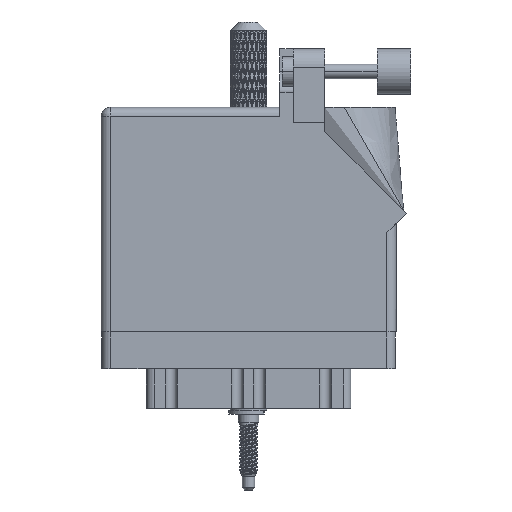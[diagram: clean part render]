
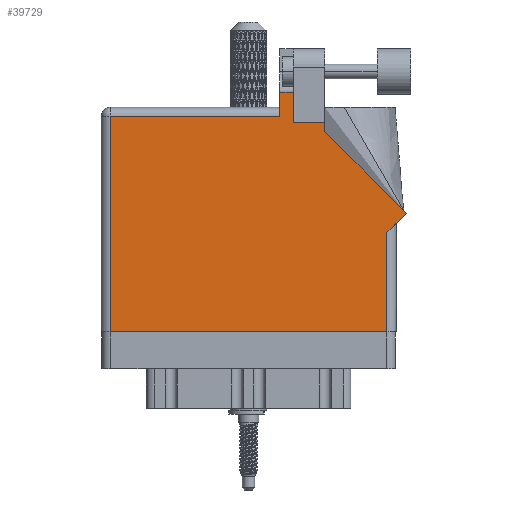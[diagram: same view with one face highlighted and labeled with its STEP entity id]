
A CAD part, front view. The second image highlights one B-rep face of the part: STEP entity #39729.
In plain terms, the highlighted face is planar.
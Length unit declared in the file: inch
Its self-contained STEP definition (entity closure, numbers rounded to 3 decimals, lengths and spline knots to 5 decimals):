
#113 = VECTOR ( 'NONE', #100295, 39.37008 ) ;
#389 = CARTESIAN_POINT ( 'NONE',  ( 1.217, 1.6315, 0. ) ) ;
#774 = ORIENTED_EDGE ( 'NONE', *, *, #37043, .T. ) ;
#975 = DIRECTION ( 'NONE',  ( 0., -1., 0. ) ) ;
#2414 = VERTEX_POINT ( 'NONE', #103825 ) ;
#4596 = ORIENTED_EDGE ( 'NONE', *, *, #92486, .T. ) ;
#6521 = VERTEX_POINT ( 'NONE', #102149 ) ;
#6803 = ORIENTED_EDGE ( 'NONE', *, *, #50928, .T. ) ;
#7591 = VERTEX_POINT ( 'NONE', #65473 ) ;
#9100 = VECTOR ( 'NONE', #975, 39.37008 ) ;
#10269 = ORIENTED_EDGE ( 'NONE', *, *, #17523, .T. ) ;
#11165 = EDGE_CURVE ( 'NONE', #44501, #67315, #84320, .T. ) ;
#11763 = CARTESIAN_POINT ( 'NONE',  ( 1.524, 1.36442, 0. ) ) ;
#12683 = FACE_OUTER_BOUND ( 'NONE', #38110, .T. ) ;
#12820 = LINE ( 'NONE', #21805, #57870 ) ;
#13620 = CARTESIAN_POINT ( 'NONE',  ( 1.217, 1.53, 0. ) ) ;
#16835 = DIRECTION ( 'NONE',  ( 0., 1., 0. ) ) ;
#17523 = EDGE_CURVE ( 'NONE', #102263, #36767, #73571, .T. ) ;
#19213 = CARTESIAN_POINT ( 'NONE',  ( 0., 1.468, 0. ) ) ;
#21202 = CARTESIAN_POINT ( 'NONE',  ( 2.01, 0.737, 0. ) ) ;
#21805 = CARTESIAN_POINT ( 'NONE',  ( 0., 0., 0. ) ) ;
#22273 = VERTEX_POINT ( 'NONE', #91431 ) ;
#22643 = VERTEX_POINT ( 'NONE', #88695 ) ;
#23249 = EDGE_CURVE ( 'NONE', #51740, #22273, #95242, .T. ) ;
#23280 = CARTESIAN_POINT ( 'NONE',  ( 2.08071, 0.80771, 0. ) ) ;
#23488 = VECTOR ( 'NONE', #25501, 39.37008 ) ;
#25501 = DIRECTION ( 'NONE',  ( -1., 0., 0. ) ) ;
#25826 = VECTOR ( 'NONE', #86325, 39.37008 ) ;
#26297 = EDGE_CURVE ( 'NONE', #6521, #51740, #90152, .T. ) ;
#29153 = CARTESIAN_POINT ( 'NONE',  ( 0.062, 0., 0. ) ) ;
#30700 = VECTOR ( 'NONE', #16835, 39.37008 ) ;
#31089 = ORIENTED_EDGE ( 'NONE', *, *, #11165, .T. ) ;
#36767 = VERTEX_POINT ( 'NONE', #29153 ) ;
#36853 = EDGE_CURVE ( 'NONE', #22643, #98463, #54058, .T. ) ;
#37043 = EDGE_CURVE ( 'NONE', #98463, #44501, #95238, .T. ) ;
#38110 = EDGE_LOOP ( 'NONE', ( #4596, #75909, #71807, #55880, #10269, #76729, #48544, #53599, #774, #31089, #6803 ) ) ;
#39729 = ADVANCED_FACE ( 'NONE', ( #12683 ), #62446, .F. ) ;
#40041 = LINE ( 'NONE', #56958, #94419 ) ;
#41007 = AXIS2_PLACEMENT_3D ( 'NONE', #78354, #86290, #94793 ) ;
#41882 = VECTOR ( 'NONE', #96271, 39.37008 ) ;
#44148 = DIRECTION ( 'NONE',  ( 0., 1., 0. ) ) ;
#44501 = VERTEX_POINT ( 'NONE', #59718 ) ;
#46687 = CARTESIAN_POINT ( 'NONE',  ( 1.524, 1.43, 0. ) ) ;
#48544 = ORIENTED_EDGE ( 'NONE', *, *, #49611, .T. ) ;
#49611 = EDGE_CURVE ( 'NONE', #7591, #22643, #104276, .T. ) ;
#50928 = EDGE_CURVE ( 'NONE', #67315, #2414, #40041, .T. ) ;
#51048 = CARTESIAN_POINT ( 'NONE',  ( 0.062, 1.468, 0. ) ) ;
#51740 = VERTEX_POINT ( 'NONE', #389 ) ;
#53599 = ORIENTED_EDGE ( 'NONE', *, *, #36853, .T. ) ;
#54058 = LINE ( 'NONE', #21202, #25826 ) ;
#54159 = DIRECTION ( 'NONE',  ( 1., 0., 0. ) ) ;
#54991 = DIRECTION ( 'NONE',  ( -0.707, 0.707, 0. ) ) ;
#54995 = DIRECTION ( 'NONE',  ( 0., -1., 0. ) ) ;
#55880 = ORIENTED_EDGE ( 'NONE', *, *, #92105, .T. ) ;
#56958 = CARTESIAN_POINT ( 'NONE',  ( 1.524, 1.43, 0. ) ) ;
#57176 = CARTESIAN_POINT ( 'NONE',  ( 0.062, 0., 0. ) ) ;
#57309 = CARTESIAN_POINT ( 'NONE',  ( 1.64177, 1.6315, 0. ) ) ;
#57870 = VECTOR ( 'NONE', #54159, 39.37008 ) ;
#58744 = EDGE_CURVE ( 'NONE', #36767, #7591, #12820, .T. ) ;
#59718 = CARTESIAN_POINT ( 'NONE',  ( 1.524, 1.36442, 0. ) ) ;
#62446 = PLANE ( 'NONE',  #41007 ) ;
#65473 = CARTESIAN_POINT ( 'NONE',  ( 1.948, 0., 0. ) ) ;
#67315 = VERTEX_POINT ( 'NONE', #46687 ) ;
#67895 = LINE ( 'NONE', #19213, #113 ) ;
#71807 = ORIENTED_EDGE ( 'NONE', *, *, #23249, .T. ) ;
#71896 = CARTESIAN_POINT ( 'NONE',  ( 1.948, 0.737, 0. ) ) ;
#73571 = LINE ( 'NONE', #57176, #9100 ) ;
#75909 = ORIENTED_EDGE ( 'NONE', *, *, #26297, .T. ) ;
#76729 = ORIENTED_EDGE ( 'NONE', *, *, #58744, .T. ) ;
#78354 = CARTESIAN_POINT ( 'NONE',  ( 0., 1.53, 0. ) ) ;
#84320 = LINE ( 'NONE', #11763, #96592 ) ;
#86290 = DIRECTION ( 'NONE',  ( 0., 0., -1. ) ) ;
#86325 = DIRECTION ( 'NONE',  ( 0.707, 0.707, 0. ) ) ;
#86665 = VECTOR ( 'NONE', #54995, 39.37008 ) ;
#88695 = CARTESIAN_POINT ( 'NONE',  ( 1.948, 0.675, 0. ) ) ;
#90152 = LINE ( 'NONE', #57309, #23488 ) ;
#91431 = CARTESIAN_POINT ( 'NONE',  ( 1.217, 1.468, 0. ) ) ;
#92105 = EDGE_CURVE ( 'NONE', #22273, #102263, #67895, .T. ) ;
#92486 = EDGE_CURVE ( 'NONE', #2414, #6521, #96895, .T. ) ;
#93678 = CARTESIAN_POINT ( 'NONE',  ( 2.08071, 0.80771, 0. ) ) ;
#94419 = VECTOR ( 'NONE', #104681, 39.37008 ) ;
#94793 = DIRECTION ( 'NONE',  ( -1., 0., 0. ) ) ;
#95238 = LINE ( 'NONE', #93678, #103676 ) ;
#95242 = LINE ( 'NONE', #13620, #86665 ) ;
#96271 = DIRECTION ( 'NONE',  ( 0., 1., 0. ) ) ;
#96592 = VECTOR ( 'NONE', #44148, 39.37008 ) ;
#96895 = LINE ( 'NONE', #104863, #30700 ) ;
#98463 = VERTEX_POINT ( 'NONE', #23280 ) ;
#100295 = DIRECTION ( 'NONE',  ( -1., 0., 0. ) ) ;
#102149 = CARTESIAN_POINT ( 'NONE',  ( 1.311, 1.6315, 0. ) ) ;
#102263 = VERTEX_POINT ( 'NONE', #51048 ) ;
#103676 = VECTOR ( 'NONE', #54991, 39.37008 ) ;
#103825 = CARTESIAN_POINT ( 'NONE',  ( 1.311, 1.43, 0. ) ) ;
#104276 = LINE ( 'NONE', #71896, #41882 ) ;
#104681 = DIRECTION ( 'NONE',  ( -1., 0., 0. ) ) ;
#104863 = CARTESIAN_POINT ( 'NONE',  ( 1.311, 1.43, 0. ) ) ;
